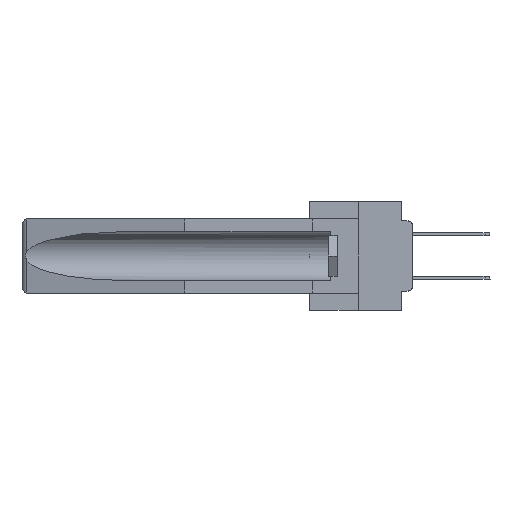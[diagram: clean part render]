
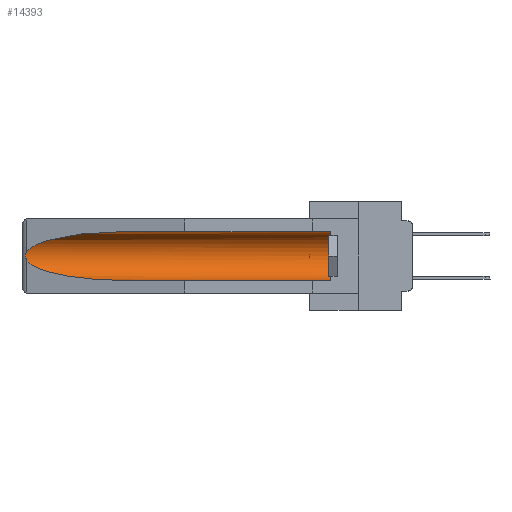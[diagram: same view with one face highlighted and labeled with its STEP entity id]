
A CAD part, left-side view. The second image highlights one B-rep face of the part: STEP entity #14393.
In plain terms, the highlighted cylindrical face has radius 2.857 mm (diameter 5.715 mm), a partial arc.
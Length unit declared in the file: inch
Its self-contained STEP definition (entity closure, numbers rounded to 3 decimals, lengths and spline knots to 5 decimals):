
#462 = VERTEX_POINT ( 'NONE', #33895 ) ;
#636 = LINE ( 'NONE', #2628, #3594 ) ;
#913 = DIRECTION ( 'NONE',  ( 0., -1., 0. ) ) ;
#1755 = ORIENTED_EDGE ( 'NONE', *, *, #32344, .T. ) ;
#2394 = CARTESIAN_POINT ( 'NONE',  ( 0.155, -0.30754, -0.1715 ) ) ;
#2454 = CARTESIAN_POINT ( 'NONE',  ( 0.26537, 1.52718, -0.19328 ) ) ;
#2628 = CARTESIAN_POINT ( 'NONE',  ( 0.155, -0.30754, -0.284 ) ) ;
#2699 = CARTESIAN_POINT ( 'NONE',  ( 0.26537, 1.52718, -0.14972 ) ) ;
#2731 = CARTESIAN_POINT ( 'NONE',  ( 0.2675, 1.53308, -0.16763 ) ) ;
#3108 =( BOUNDED_CURVE ( )  B_SPLINE_CURVE ( 3, ( #16114, #9715, #37939, #35073 ),
 .UNSPECIFIED., .F., .F. ) 
 B_SPLINE_CURVE_WITH_KNOTS ( ( 4, 4 ),
 ( 4.71239, 6.08839 ),
 .UNSPECIFIED. ) 
 CURVE ( )  GEOMETRIC_REPRESENTATION_ITEM ( )  RATIONAL_B_SPLINE_CURVE ( ( 1., 0.848, 0.848, 1. ) ) 
 REPRESENTATION_ITEM ( '' )  );
#3594 = VECTOR ( 'NONE', #36595, 39.37008 ) ;
#4340 = EDGE_CURVE ( 'NONE', #32758, #462, #17116, .T. ) ;
#5031 = CIRCLE ( 'NONE', #23560, 0.1125 ) ;
#5481 = CARTESIAN_POINT ( 'NONE',  ( 0.26654, 1.53092, -0.15636 ) ) ;
#5873 = CARTESIAN_POINT ( 'NONE',  ( 0.2675, 1.53308, -0.17534 ) ) ;
#6734 = EDGE_CURVE ( 'NONE', #37297, #20476, #636, .T. ) ;
#7058 = DIRECTION ( 'NONE',  ( 0., 0., 1. ) ) ;
#8159 = CARTESIAN_POINT ( 'NONE',  ( 0.155, -0.30754, -0.059 ) ) ;
#9102 = DIRECTION ( 'NONE',  ( 0., 0., 1. ) ) ;
#9715 = CARTESIAN_POINT ( 'NONE',  ( 0.21114, 1.30732, -0.059 ) ) ;
#10001 = ORIENTED_EDGE ( 'NONE', *, *, #6734, .F. ) ;
#10620 = CARTESIAN_POINT ( 'NONE',  ( 0.155, 0.126, -0.1715 ) ) ;
#11137 = ORIENTED_EDGE ( 'NONE', *, *, #4340, .T. ) ;
#13826 = CARTESIAN_POINT ( 'NONE',  ( 0.155, 0.126, -0.059 ) ) ;
#14393 = ADVANCED_FACE ( 'NONE', ( #29865 ), #17538, .F. ) ;
#14741 = CARTESIAN_POINT ( 'NONE',  ( 0.26597, 1.52961, -0.15275 ) ) ;
#15093 = CARTESIAN_POINT ( 'NONE',  ( 0.26537, 1.52718, -0.19328 ) ) ;
#15160 = CARTESIAN_POINT ( 'NONE',  ( 0.2673, 1.5327, -0.16383 ) ) ;
#15817 = EDGE_CURVE ( 'NONE', #22943, #19726, #31269, .T. ) ;
#15959 = VECTOR ( 'NONE', #33099, 39.37008 ) ;
#16114 = CARTESIAN_POINT ( 'NONE',  ( 0.155, 1.07973, -0.059 ) ) ;
#16480 = EDGE_LOOP ( 'NONE', ( #39463, #11137, #17786, #10001, #1755, #34327 ) ) ;
#16571 = CARTESIAN_POINT ( 'NONE',  ( 0.155, 1.07973, -0.059 ) ) ;
#16862 = AXIS2_PLACEMENT_3D ( 'NONE', #2394, #27455, #9102 ) ;
#17116 = B_SPLINE_CURVE_WITH_KNOTS ( 'NONE', 3,
 ( #33982, #14741, #5481, #15160, #2731, #5873, #27377, #30577, #21160, #2454 ),
 .UNSPECIFIED., .F., .F.,
 ( 4, 2, 2, 2, 4 ),
 ( 0., 0.00029, 0.00058, 0.00087, 0.00117 ),
 .UNSPECIFIED. ) ;
#17538 = CYLINDRICAL_SURFACE ( 'NONE', #16862, 0.1125 ) ;
#17786 = ORIENTED_EDGE ( 'NONE', *, *, #18513, .T. ) ;
#18513 = EDGE_CURVE ( 'NONE', #462, #20476, #37746, .T. ) ;
#18859 = CARTESIAN_POINT ( 'NONE',  ( 0.155, 1.07973, -0.284 ) ) ;
#19726 = VERTEX_POINT ( 'NONE', #16571 ) ;
#20476 = VERTEX_POINT ( 'NONE', #34946 ) ;
#21160 = CARTESIAN_POINT ( 'NONE',  ( 0.26597, 1.5296, -0.19026 ) ) ;
#21437 = CARTESIAN_POINT ( 'NONE',  ( 0.155, 0.126, -0.284 ) ) ;
#22943 = VERTEX_POINT ( 'NONE', #13826 ) ;
#23560 = AXIS2_PLACEMENT_3D ( 'NONE', #10620, #913, #7058 ) ;
#25190 = CARTESIAN_POINT ( 'NONE',  ( 0.21114, 1.30732, -0.284 ) ) ;
#27377 = CARTESIAN_POINT ( 'NONE',  ( 0.2673, 1.53269, -0.17917 ) ) ;
#27455 = DIRECTION ( 'NONE',  ( 0., 1., 0. ) ) ;
#29865 = FACE_OUTER_BOUND ( 'NONE', #16480, .T. ) ;
#29920 = EDGE_CURVE ( 'NONE', #19726, #32758, #3108, .T. ) ;
#30577 = CARTESIAN_POINT ( 'NONE',  ( 0.26655, 1.53094, -0.18657 ) ) ;
#31269 = LINE ( 'NONE', #8159, #15959 ) ;
#32344 = EDGE_CURVE ( 'NONE', #37297, #22943, #5031, .T. ) ;
#32758 = VERTEX_POINT ( 'NONE', #2699 ) ;
#33099 = DIRECTION ( 'NONE',  ( 0., 1., 0. ) ) ;
#33895 = CARTESIAN_POINT ( 'NONE',  ( 0.26537, 1.52718, -0.19328 ) ) ;
#33982 = CARTESIAN_POINT ( 'NONE',  ( 0.26537, 1.52718, -0.14972 ) ) ;
#34327 = ORIENTED_EDGE ( 'NONE', *, *, #15817, .T. ) ;
#34555 = CARTESIAN_POINT ( 'NONE',  ( 0.25451, 1.48313, -0.24835 ) ) ;
#34946 = CARTESIAN_POINT ( 'NONE',  ( 0.155, 1.07973, -0.284 ) ) ;
#35073 = CARTESIAN_POINT ( 'NONE',  ( 0.26537, 1.52718, -0.14972 ) ) ;
#36595 = DIRECTION ( 'NONE',  ( 0., 1., 0. ) ) ;
#37297 = VERTEX_POINT ( 'NONE', #21437 ) ;
#37746 =( BOUNDED_CURVE ( )  B_SPLINE_CURVE ( 3, ( #15093, #34555, #25190, #18859 ),
 .UNSPECIFIED., .F., .F. ) 
 B_SPLINE_CURVE_WITH_KNOTS ( ( 4, 4 ),
 ( 0.1948, 1.5708 ),
 .UNSPECIFIED. ) 
 CURVE ( )  GEOMETRIC_REPRESENTATION_ITEM ( )  RATIONAL_B_SPLINE_CURVE ( ( 1., 0.848, 0.848, 1. ) ) 
 REPRESENTATION_ITEM ( '' )  );
#37939 = CARTESIAN_POINT ( 'NONE',  ( 0.25451, 1.48313, -0.09465 ) ) ;
#39463 = ORIENTED_EDGE ( 'NONE', *, *, #29920, .T. ) ;
